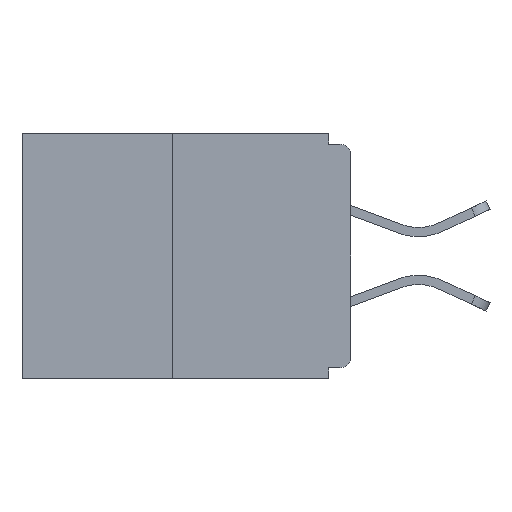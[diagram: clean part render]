
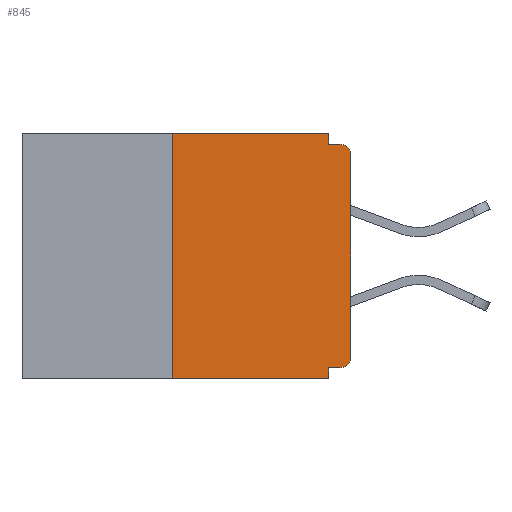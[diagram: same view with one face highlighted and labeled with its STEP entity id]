
A CAD part, left-side view. The second image highlights one B-rep face of the part: STEP entity #845.
In plain terms, the highlighted planar face has unit normal (-1, 0, 0).
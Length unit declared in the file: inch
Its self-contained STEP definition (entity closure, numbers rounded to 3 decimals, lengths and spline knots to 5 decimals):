
#540 = EDGE_CURVE ( 'NONE', #21015, #15310, #4825, .T. ) ;
#845 = ADVANCED_FACE ( 'NONE', ( #23547 ), #15694, .F. ) ;
#1215 = LINE ( 'NONE', #21756, #23902 ) ;
#1459 = ORIENTED_EDGE ( 'NONE', *, *, #21532, .T. ) ;
#2342 = VECTOR ( 'NONE', #24650, 39.37008 ) ;
#2465 = ORIENTED_EDGE ( 'NONE', *, *, #9435, .F. ) ;
#2985 = LINE ( 'NONE', #16063, #2342 ) ;
#3144 = ORIENTED_EDGE ( 'NONE', *, *, #25118, .F. ) ;
#3422 = LINE ( 'NONE', #20296, #17403 ) ;
#4168 = VERTEX_POINT ( 'NONE', #9560 ) ;
#4565 = LINE ( 'NONE', #10799, #8596 ) ;
#4594 = DIRECTION ( 'NONE',  ( -1., 0., 0. ) ) ;
#4746 = LINE ( 'NONE', #17312, #18049 ) ;
#4825 = LINE ( 'NONE', #5158, #20822 ) ;
#5158 = CARTESIAN_POINT ( 'NONE',  ( 0., 0.031, -0.343 ) ) ;
#5362 = DIRECTION ( 'NONE',  ( 0., 0., -1. ) ) ;
#5443 = DIRECTION ( 'NONE',  ( -1., 0., 0. ) ) ;
#6404 = ORIENTED_EDGE ( 'NONE', *, *, #17191, .F. ) ;
#6597 = EDGE_CURVE ( 'NONE', #8359, #14084, #4565, .T. ) ;
#7309 = DIRECTION ( 'NONE',  ( 0., 0., -1. ) ) ;
#7489 = VERTEX_POINT ( 'NONE', #13234 ) ;
#8271 = CARTESIAN_POINT ( 'NONE',  ( 0., 0.46, -0.343 ) ) ;
#8289 = CARTESIAN_POINT ( 'NONE',  ( 0., 0.031, -0.343 ) ) ;
#8359 = VERTEX_POINT ( 'NONE', #12102 ) ;
#8596 = VECTOR ( 'NONE', #9016, 39.37008 ) ;
#8627 = VERTEX_POINT ( 'NONE', #25888 ) ;
#8814 = DIRECTION ( 'NONE',  ( 0., 1., 0. ) ) ;
#9016 = DIRECTION ( 'NONE',  ( 0., 0., 1. ) ) ;
#9104 = DIRECTION ( 'NONE',  ( 0., -1., 0. ) ) ;
#9435 = EDGE_CURVE ( 'NONE', #14175, #8627, #1215, .T. ) ;
#9484 = LINE ( 'NONE', #19319, #23142 ) ;
#9560 = CARTESIAN_POINT ( 'NONE',  ( 0., 0.25, 0. ) ) ;
#9698 = EDGE_LOOP ( 'NONE', ( #3144, #19128, #11419, #24375, #6404, #1459, #15770, #11108, #2465, #12147 ) ) ;
#10799 = CARTESIAN_POINT ( 'NONE',  ( 0., 0., 0. ) ) ;
#11108 = ORIENTED_EDGE ( 'NONE', *, *, #22950, .T. ) ;
#11419 = ORIENTED_EDGE ( 'NONE', *, *, #27533, .T. ) ;
#11849 = EDGE_CURVE ( 'NONE', #19416, #4168, #3422, .T. ) ;
#11912 = LINE ( 'NONE', #8271, #16905 ) ;
#12102 = CARTESIAN_POINT ( 'NONE',  ( 0., 0., -0.313 ) ) ;
#12147 = ORIENTED_EDGE ( 'NONE', *, *, #20556, .F. ) ;
#12350 = DIRECTION ( 'NONE',  ( 0., -1., 0. ) ) ;
#12587 = AXIS2_PLACEMENT_3D ( 'NONE', #22224, #5443, #20312 ) ;
#13184 = CIRCLE ( 'NONE', #14576, 0.015 ) ;
#13234 = CARTESIAN_POINT ( 'NONE',  ( 0., 0.031, 0. ) ) ;
#13283 = CIRCLE ( 'NONE', #12587, 0.015 ) ;
#13346 = VERTEX_POINT ( 'NONE', #16901 ) ;
#14084 = VERTEX_POINT ( 'NONE', #18322 ) ;
#14175 = VERTEX_POINT ( 'NONE', #20938 ) ;
#14576 = AXIS2_PLACEMENT_3D ( 'NONE', #21450, #4594, #21355 ) ;
#14775 = CARTESIAN_POINT ( 'NONE',  ( 0., 0.031, -0.328 ) ) ;
#15310 = VERTEX_POINT ( 'NONE', #8289 ) ;
#15694 = PLANE ( 'NONE',  #23771 ) ;
#15770 = ORIENTED_EDGE ( 'NONE', *, *, #6597, .T. ) ;
#15868 = CARTESIAN_POINT ( 'NONE',  ( 0., 0.46, 0. ) ) ;
#16063 = CARTESIAN_POINT ( 'NONE',  ( 0., 0.031, 0. ) ) ;
#16088 = CARTESIAN_POINT ( 'NONE',  ( 0., 0.25, -0.343 ) ) ;
#16901 = CARTESIAN_POINT ( 'NONE',  ( 0., 0.015, -0.328 ) ) ;
#16905 = VECTOR ( 'NONE', #12350, 39.37008 ) ;
#17191 = EDGE_CURVE ( 'NONE', #13346, #21015, #4746, .T. ) ;
#17312 = CARTESIAN_POINT ( 'NONE',  ( 0., 0., -0.328 ) ) ;
#17403 = VECTOR ( 'NONE', #26520, 39.37008 ) ;
#18049 = VECTOR ( 'NONE', #8814, 39.37008 ) ;
#18322 = CARTESIAN_POINT ( 'NONE',  ( 0., 0., -0.03 ) ) ;
#19128 = ORIENTED_EDGE ( 'NONE', *, *, #11849, .F. ) ;
#19319 = CARTESIAN_POINT ( 'NONE',  ( 0., 0.46, 0. ) ) ;
#19416 = VERTEX_POINT ( 'NONE', #16088 ) ;
#20296 = CARTESIAN_POINT ( 'NONE',  ( 0., 0.25, 0. ) ) ;
#20312 = DIRECTION ( 'NONE',  ( 0., 0., -1. ) ) ;
#20556 = EDGE_CURVE ( 'NONE', #7489, #14175, #2985, .T. ) ;
#20822 = VECTOR ( 'NONE', #7309, 39.37008 ) ;
#20938 = CARTESIAN_POINT ( 'NONE',  ( 0., 0.031, -0.015 ) ) ;
#21015 = VERTEX_POINT ( 'NONE', #14775 ) ;
#21355 = DIRECTION ( 'NONE',  ( 0., 0., -1. ) ) ;
#21450 = CARTESIAN_POINT ( 'NONE',  ( 0., 0.015, -0.03 ) ) ;
#21491 = DIRECTION ( 'NONE',  ( 0., -1., 0. ) ) ;
#21532 = EDGE_CURVE ( 'NONE', #13346, #8359, #13283, .T. ) ;
#21756 = CARTESIAN_POINT ( 'NONE',  ( 0., 0., -0.015 ) ) ;
#22224 = CARTESIAN_POINT ( 'NONE',  ( 0., 0.015, -0.313 ) ) ;
#22950 = EDGE_CURVE ( 'NONE', #14084, #8627, #13184, .T. ) ;
#23142 = VECTOR ( 'NONE', #21491, 39.37008 ) ;
#23547 = FACE_OUTER_BOUND ( 'NONE', #9698, .T. ) ;
#23771 = AXIS2_PLACEMENT_3D ( 'NONE', #15868, #24279, #5362 ) ;
#23902 = VECTOR ( 'NONE', #9104, 39.37008 ) ;
#24279 = DIRECTION ( 'NONE',  ( 1., 0., 0. ) ) ;
#24375 = ORIENTED_EDGE ( 'NONE', *, *, #540, .F. ) ;
#24650 = DIRECTION ( 'NONE',  ( 0., 0., -1. ) ) ;
#25118 = EDGE_CURVE ( 'NONE', #4168, #7489, #9484, .T. ) ;
#25888 = CARTESIAN_POINT ( 'NONE',  ( 0., 0.015, -0.015 ) ) ;
#26520 = DIRECTION ( 'NONE',  ( 0., 0., 1. ) ) ;
#27533 = EDGE_CURVE ( 'NONE', #19416, #15310, #11912, .T. ) ;
